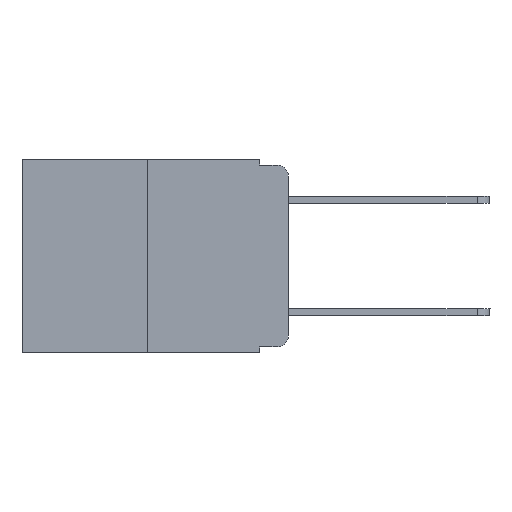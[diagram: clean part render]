
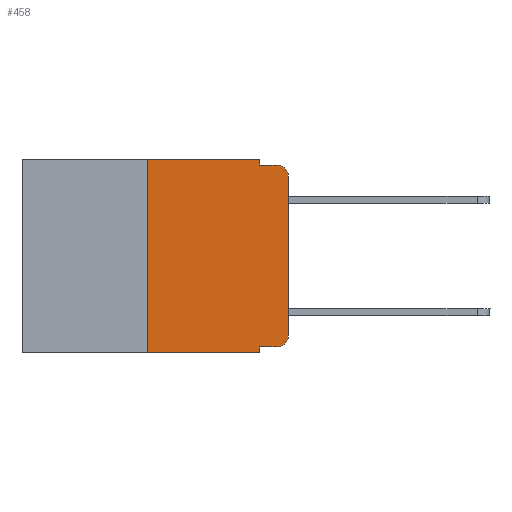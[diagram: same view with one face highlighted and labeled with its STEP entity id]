
A CAD part, left-side view. The second image highlights one B-rep face of the part: STEP entity #458.
In plain terms, the highlighted planar face has unit normal (-1, 0, 0).
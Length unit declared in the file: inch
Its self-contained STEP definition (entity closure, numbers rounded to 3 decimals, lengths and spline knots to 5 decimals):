
#54 = VERTEX_POINT ( 'NONE', #4777 ) ;
#426 = DIRECTION ( 'NONE',  ( 0., -1., 0. ) ) ;
#431 = CARTESIAN_POINT ( 'NONE',  ( 0., 0.25, 0. ) ) ;
#458 = ADVANCED_FACE ( 'NONE', ( #6380 ), #9650, .F. ) ;
#676 = CIRCLE ( 'NONE', #2042, 0.02 ) ;
#758 = VERTEX_POINT ( 'NONE', #6900 ) ;
#1346 = CARTESIAN_POINT ( 'NONE',  ( 0., 0.02, -0.03 ) ) ;
#1468 = DIRECTION ( 'NONE',  ( 0., 0., 1. ) ) ;
#1615 = VERTEX_POINT ( 'NONE', #431 ) ;
#1759 = LINE ( 'NONE', #7416, #5875 ) ;
#1819 = VECTOR ( 'NONE', #2398, 39.37008 ) ;
#1885 = CARTESIAN_POINT ( 'NONE',  ( 0., 0.051, -0.333 ) ) ;
#2035 = VERTEX_POINT ( 'NONE', #3603 ) ;
#2042 = AXIS2_PLACEMENT_3D ( 'NONE', #1346, #7972, #3772 ) ;
#2154 = CIRCLE ( 'NONE', #8953, 0.02 ) ;
#2166 = VECTOR ( 'NONE', #2238, 39.37008 ) ;
#2193 = EDGE_CURVE ( 'NONE', #1615, #2035, #6524, .T. ) ;
#2238 = DIRECTION ( 'NONE',  ( 0., -1., 0. ) ) ;
#2398 = DIRECTION ( 'NONE',  ( 0., -1., 0. ) ) ;
#2498 = EDGE_CURVE ( 'NONE', #758, #1615, #9561, .T. ) ;
#2716 = CARTESIAN_POINT ( 'NONE',  ( 0., 0.02, -0.313 ) ) ;
#2793 = ORIENTED_EDGE ( 'NONE', *, *, #3658, .T. ) ;
#2836 = LINE ( 'NONE', #9211, #6522 ) ;
#2965 = ORIENTED_EDGE ( 'NONE', *, *, #7073, .F. ) ;
#3603 = CARTESIAN_POINT ( 'NONE',  ( 0., 0.051, 0. ) ) ;
#3653 = VECTOR ( 'NONE', #1468, 39.37008 ) ;
#3658 = EDGE_CURVE ( 'NONE', #4284, #6278, #2154, .T. ) ;
#3668 = DIRECTION ( 'NONE',  ( -1., 0., 0. ) ) ;
#3772 = DIRECTION ( 'NONE',  ( 0., 0., -1. ) ) ;
#3777 = EDGE_CURVE ( 'NONE', #54, #7612, #676, .T. ) ;
#4131 = CARTESIAN_POINT ( 'NONE',  ( 0., 0., 0. ) ) ;
#4202 = CARTESIAN_POINT ( 'NONE',  ( 0., 0.473, 0. ) ) ;
#4284 = VERTEX_POINT ( 'NONE', #6919 ) ;
#4496 = CARTESIAN_POINT ( 'NONE',  ( 0., 0.051, -0.333 ) ) ;
#4560 = VECTOR ( 'NONE', #4712, 39.37008 ) ;
#4606 = ORIENTED_EDGE ( 'NONE', *, *, #3777, .T. ) ;
#4712 = DIRECTION ( 'NONE',  ( 0., -1., 0. ) ) ;
#4720 = VERTEX_POINT ( 'NONE', #7061 ) ;
#4777 = CARTESIAN_POINT ( 'NONE',  ( 0., 0., -0.03 ) ) ;
#4826 = LINE ( 'NONE', #4933, #1819 ) ;
#4933 = CARTESIAN_POINT ( 'NONE',  ( 0., 0.473, -0.343 ) ) ;
#5143 = EDGE_CURVE ( 'NONE', #6278, #54, #5868, .T. ) ;
#5194 = ORIENTED_EDGE ( 'NONE', *, *, #2498, .F. ) ;
#5317 = DIRECTION ( 'NONE',  ( 0., 0., 1. ) ) ;
#5365 = ORIENTED_EDGE ( 'NONE', *, *, #8010, .T. ) ;
#5408 = VECTOR ( 'NONE', #5317, 39.37008 ) ;
#5416 = ORIENTED_EDGE ( 'NONE', *, *, #7757, .T. ) ;
#5865 = AXIS2_PLACEMENT_3D ( 'NONE', #7337, #8962, #8104 ) ;
#5868 = LINE ( 'NONE', #4131, #3653 ) ;
#5874 = DIRECTION ( 'NONE',  ( 0., 0., -1. ) ) ;
#5875 = VECTOR ( 'NONE', #7310, 39.37008 ) ;
#5955 = CARTESIAN_POINT ( 'NONE',  ( 0., 0.051, -0.343 ) ) ;
#6127 = CARTESIAN_POINT ( 'NONE',  ( 0., 0.051, -0.01 ) ) ;
#6278 = VERTEX_POINT ( 'NONE', #6838 ) ;
#6380 = FACE_OUTER_BOUND ( 'NONE', #10339, .T. ) ;
#6522 = VECTOR ( 'NONE', #8371, 39.37008 ) ;
#6524 = LINE ( 'NONE', #4202, #4560 ) ;
#6716 = VERTEX_POINT ( 'NONE', #1885 ) ;
#6838 = CARTESIAN_POINT ( 'NONE',  ( 0., 0., -0.313 ) ) ;
#6867 = LINE ( 'NONE', #4496, #2166 ) ;
#6900 = CARTESIAN_POINT ( 'NONE',  ( 0., 0.25, -0.343 ) ) ;
#6919 = CARTESIAN_POINT ( 'NONE',  ( 0., 0.02, -0.333 ) ) ;
#7061 = CARTESIAN_POINT ( 'NONE',  ( 0., 0.051, -0.01 ) ) ;
#7073 = EDGE_CURVE ( 'NONE', #6716, #8415, #2836, .T. ) ;
#7294 = ORIENTED_EDGE ( 'NONE', *, *, #2193, .F. ) ;
#7310 = DIRECTION ( 'NONE',  ( 0., 0., -1. ) ) ;
#7333 = ORIENTED_EDGE ( 'NONE', *, *, #5143, .T. ) ;
#7337 = CARTESIAN_POINT ( 'NONE',  ( 0., 0.473, 0. ) ) ;
#7416 = CARTESIAN_POINT ( 'NONE',  ( 0., 0.051, 0. ) ) ;
#7557 = VECTOR ( 'NONE', #426, 39.37008 ) ;
#7612 = VERTEX_POINT ( 'NONE', #8733 ) ;
#7676 = LINE ( 'NONE', #6127, #7557 ) ;
#7679 = ORIENTED_EDGE ( 'NONE', *, *, #9172, .F. ) ;
#7757 = EDGE_CURVE ( 'NONE', #758, #8415, #4826, .T. ) ;
#7972 = DIRECTION ( 'NONE',  ( -1., 0., 0. ) ) ;
#8010 = EDGE_CURVE ( 'NONE', #6716, #4284, #6867, .T. ) ;
#8067 = EDGE_CURVE ( 'NONE', #4720, #7612, #7676, .T. ) ;
#8104 = DIRECTION ( 'NONE',  ( 0., 0., -1. ) ) ;
#8371 = DIRECTION ( 'NONE',  ( 0., 0., -1. ) ) ;
#8415 = VERTEX_POINT ( 'NONE', #5955 ) ;
#8733 = CARTESIAN_POINT ( 'NONE',  ( 0., 0.02, -0.01 ) ) ;
#8953 = AXIS2_PLACEMENT_3D ( 'NONE', #2716, #3668, #5874 ) ;
#8962 = DIRECTION ( 'NONE',  ( 1., 0., 0. ) ) ;
#9172 = EDGE_CURVE ( 'NONE', #2035, #4720, #1759, .T. ) ;
#9211 = CARTESIAN_POINT ( 'NONE',  ( 0., 0.051, 0. ) ) ;
#9509 = ORIENTED_EDGE ( 'NONE', *, *, #8067, .F. ) ;
#9512 = CARTESIAN_POINT ( 'NONE',  ( 0., 0.25, 0. ) ) ;
#9561 = LINE ( 'NONE', #9512, #5408 ) ;
#9650 = PLANE ( 'NONE',  #5865 ) ;
#10339 = EDGE_LOOP ( 'NONE', ( #7333, #4606, #9509, #7679, #7294, #5194, #5416, #2965, #5365, #2793 ) ) ;
